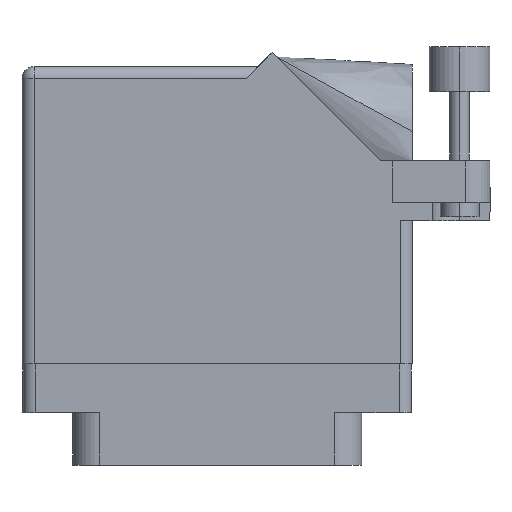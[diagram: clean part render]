
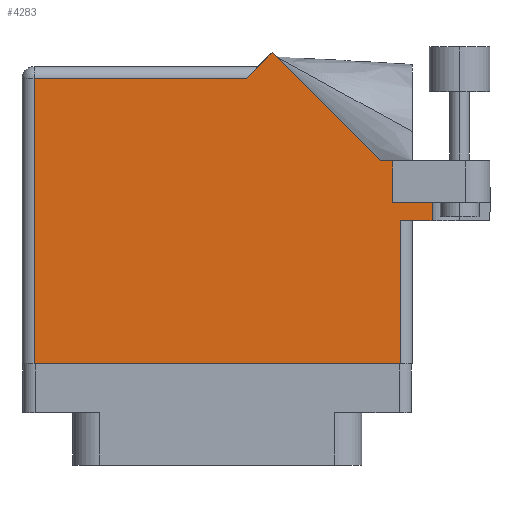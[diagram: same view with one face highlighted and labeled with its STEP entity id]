
A CAD part, front view. The second image highlights one B-rep face of the part: STEP entity #4283.
In plain terms, the highlighted face is planar.
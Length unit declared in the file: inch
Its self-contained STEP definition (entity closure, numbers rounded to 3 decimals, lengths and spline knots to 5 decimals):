
#111 = LINE ( 'NONE', #15720, #35841 ) ;
#513 = LINE ( 'NONE', #24102, #22114 ) ;
#809 = CARTESIAN_POINT ( 'NONE',  ( 0.28271, 1.50071, 0.455 ) ) ;
#1382 = VECTOR ( 'NONE', #35813, 39.37008 ) ;
#1389 = ORIENTED_EDGE ( 'NONE', *, *, #30777, .T. ) ;
#2406 = ORIENTED_EDGE ( 'NONE', *, *, #34366, .F. ) ;
#2765 = DIRECTION ( 'NONE',  ( -0.707, 0.707, 0. ) ) ;
#4138 = DIRECTION ( 'NONE',  ( -0.707, -0.707, 0. ) ) ;
#4283 = ADVANCED_FACE ( 'NONE', ( #11215 ), #12087, .F. ) ;
#4324 = EDGE_CURVE ( 'NONE', #29148, #31012, #14717, .T. ) ;
#4490 = ORIENTED_EDGE ( 'NONE', *, *, #19827, .T. ) ;
#4820 = CARTESIAN_POINT ( 'NONE',  ( 0.83942, 0.944, 0.455 ) ) ;
#4912 = DIRECTION ( 'NONE',  ( 1., 0., 0. ) ) ;
#5015 = VERTEX_POINT ( 'NONE', #12479 ) ;
#5764 = CARTESIAN_POINT ( 'NONE',  ( 0.943, 0.637, 0.455 ) ) ;
#6365 = ORIENTED_EDGE ( 'NONE', *, *, #27924, .T. ) ;
#6438 = DIRECTION ( 'NONE',  ( 0., 0., -1. ) ) ;
#6688 = CARTESIAN_POINT ( 'NONE',  ( -1.005, 1.43, 0.455 ) ) ;
#6884 = VECTOR ( 'NONE', #4138, 39.37008 ) ;
#7069 = EDGE_CURVE ( 'NONE', #5015, #29148, #513, .T. ) ;
#7101 = CARTESIAN_POINT ( 'NONE',  ( -0.943, -0.1, 0.455 ) ) ;
#7248 = VECTOR ( 'NONE', #12599, 39.37008 ) ;
#7320 = VECTOR ( 'NONE', #35519, 39.37008 ) ;
#7758 = DIRECTION ( 'NONE',  ( 0., 1., 0. ) ) ;
#8107 = CARTESIAN_POINT ( 'NONE',  ( -0.943, 1.368, 0.455 ) ) ;
#8108 = VECTOR ( 'NONE', #2765, 39.37008 ) ;
#8667 = CARTESIAN_POINT ( 'NONE',  ( 0.83942, 0.944, 0.455 ) ) ;
#8926 = ORIENTED_EDGE ( 'NONE', *, *, #4324, .T. ) ;
#8947 = VERTEX_POINT ( 'NONE', #9683 ) ;
#9683 = CARTESIAN_POINT ( 'NONE',  ( 0.905, 0.731, 0.455 ) ) ;
#9856 = DIRECTION ( 'NONE',  ( -1., 0., 0. ) ) ;
#10146 = LINE ( 'NONE', #32257, #32215 ) ;
#10285 = ORIENTED_EDGE ( 'NONE', *, *, #22574, .T. ) ;
#10416 = LINE ( 'NONE', #35432, #6884 ) ;
#10838 = CARTESIAN_POINT ( 'NONE',  ( 0.905, 0.731, 0.455 ) ) ;
#11215 = FACE_OUTER_BOUND ( 'NONE', #20851, .T. ) ;
#12087 = PLANE ( 'NONE',  #19254 ) ;
#12090 = LINE ( 'NONE', #10838, #27983 ) ;
#12479 = CARTESIAN_POINT ( 'NONE',  ( 0.943, -0.1, 0.455 ) ) ;
#12495 = CARTESIAN_POINT ( 'NONE',  ( 0.15, 1.368, 0.455 ) ) ;
#12599 = DIRECTION ( 'NONE',  ( 1., 0., 0. ) ) ;
#12626 = LINE ( 'NONE', #15642, #7320 ) ;
#12815 = CARTESIAN_POINT ( 'NONE',  ( -1.005, 1.368, 0.455 ) ) ;
#13127 = VERTEX_POINT ( 'NONE', #12495 ) ;
#13885 = ORIENTED_EDGE ( 'NONE', *, *, #36133, .T. ) ;
#14717 = LINE ( 'NONE', #34805, #7248 ) ;
#14900 = LINE ( 'NONE', #12815, #18855 ) ;
#15483 = DIRECTION ( 'NONE',  ( 1., 0., 0. ) ) ;
#15591 = LINE ( 'NONE', #8667, #8108 ) ;
#15642 = CARTESIAN_POINT ( 'NONE',  ( 1.1065, 1.06177, 0.455 ) ) ;
#15720 = CARTESIAN_POINT ( 'NONE',  ( -1.005, -0.1, 0.455 ) ) ;
#18570 = ORIENTED_EDGE ( 'NONE', *, *, #27158, .T. ) ;
#18855 = VECTOR ( 'NONE', #9856, 39.37008 ) ;
#19254 = AXIS2_PLACEMENT_3D ( 'NONE', #6688, #6438, #23558 ) ;
#19581 = CARTESIAN_POINT ( 'NONE',  ( 1.1065, 0.637, 0.455 ) ) ;
#19827 = EDGE_CURVE ( 'NONE', #23772, #5015, #111, .T. ) ;
#20851 = EDGE_LOOP ( 'NONE', ( #4490, #35775, #8926, #33889, #2406, #6365, #1389, #10285, #18570, #13885, #22923 ) ) ;
#21161 = CARTESIAN_POINT ( 'NONE',  ( -0.943, -0.1, 0.455 ) ) ;
#21176 = EDGE_CURVE ( 'NONE', #28714, #31012, #12626, .T. ) ;
#21727 = LINE ( 'NONE', #21161, #27025 ) ;
#22114 = VECTOR ( 'NONE', #32861, 39.37008 ) ;
#22574 = EDGE_CURVE ( 'NONE', #27847, #32287, #15591, .T. ) ;
#22923 = ORIENTED_EDGE ( 'NONE', *, *, #28898, .T. ) ;
#23558 = DIRECTION ( 'NONE',  ( -1., 0., 0. ) ) ;
#23772 = VERTEX_POINT ( 'NONE', #7101 ) ;
#24102 = CARTESIAN_POINT ( 'NONE',  ( 0.943, 0.637, 0.455 ) ) ;
#25239 = VERTEX_POINT ( 'NONE', #8107 ) ;
#25562 = VERTEX_POINT ( 'NONE', #25828 ) ;
#25828 = CARTESIAN_POINT ( 'NONE',  ( 0.905, 0.944, 0.455 ) ) ;
#26473 = CARTESIAN_POINT ( 'NONE',  ( 1.1065, 0.731, 0.455 ) ) ;
#26930 = LINE ( 'NONE', #32977, #1382 ) ;
#27025 = VECTOR ( 'NONE', #32769, 39.37008 ) ;
#27158 = EDGE_CURVE ( 'NONE', #32287, #13127, #10416, .T. ) ;
#27847 = VERTEX_POINT ( 'NONE', #4820 ) ;
#27924 = EDGE_CURVE ( 'NONE', #8947, #25562, #12090, .T. ) ;
#27983 = VECTOR ( 'NONE', #7758, 39.37008 ) ;
#28714 = VERTEX_POINT ( 'NONE', #26473 ) ;
#28898 = EDGE_CURVE ( 'NONE', #25239, #23772, #21727, .T. ) ;
#29148 = VERTEX_POINT ( 'NONE', #5764 ) ;
#30777 = EDGE_CURVE ( 'NONE', #25562, #27847, #26930, .T. ) ;
#31012 = VERTEX_POINT ( 'NONE', #19581 ) ;
#32215 = VECTOR ( 'NONE', #15483, 39.37008 ) ;
#32257 = CARTESIAN_POINT ( 'NONE',  ( 0.905, 0.731, 0.455 ) ) ;
#32287 = VERTEX_POINT ( 'NONE', #809 ) ;
#32769 = DIRECTION ( 'NONE',  ( 0., -1., 0. ) ) ;
#32861 = DIRECTION ( 'NONE',  ( 0., 1., 0. ) ) ;
#32977 = CARTESIAN_POINT ( 'NONE',  ( 1.405, 0.944, 0.455 ) ) ;
#33889 = ORIENTED_EDGE ( 'NONE', *, *, #21176, .F. ) ;
#34366 = EDGE_CURVE ( 'NONE', #8947, #28714, #10146, .T. ) ;
#34805 = CARTESIAN_POINT ( 'NONE',  ( 1.005, 0.637, 0.455 ) ) ;
#35432 = CARTESIAN_POINT ( 'NONE',  ( 0.212, 1.43, 0.455 ) ) ;
#35519 = DIRECTION ( 'NONE',  ( 0., -1., 0. ) ) ;
#35775 = ORIENTED_EDGE ( 'NONE', *, *, #7069, .T. ) ;
#35813 = DIRECTION ( 'NONE',  ( -1., 0., 0. ) ) ;
#35841 = VECTOR ( 'NONE', #4912, 39.37008 ) ;
#36133 = EDGE_CURVE ( 'NONE', #13127, #25239, #14900, .T. ) ;
